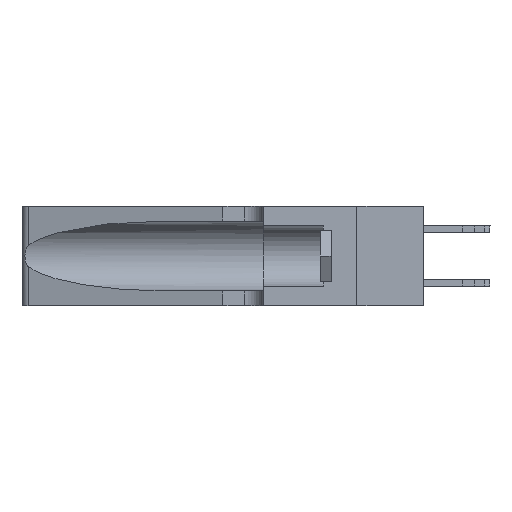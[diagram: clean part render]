
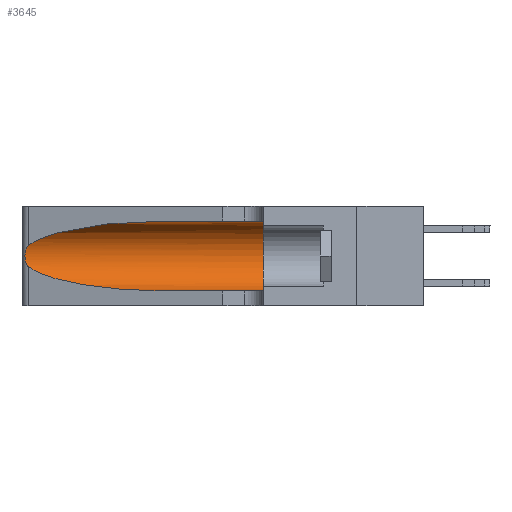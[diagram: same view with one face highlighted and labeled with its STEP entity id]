
A CAD part, left-side view. The second image highlights one B-rep face of the part: STEP entity #3645.
In plain terms, the highlighted cylindrical face has radius 3.308 mm (diameter 6.617 mm), a partial arc.
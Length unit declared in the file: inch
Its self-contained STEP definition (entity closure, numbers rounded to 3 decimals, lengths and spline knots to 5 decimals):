
#310 = AXIS2_PLACEMENT_3D ( 'NONE', #10544, #16618, #24730 ) ;
#458 = CARTESIAN_POINT ( 'NONE',  ( 0.1305, 1.61858, 0.185 ) ) ;
#866 = ORIENTED_EDGE ( 'NONE', *, *, #23540, .T. ) ;
#966 = ORIENTED_EDGE ( 'NONE', *, *, #2103, .T. ) ;
#1143 = DIRECTION ( 'NONE',  ( 0., -1., 0. ) ) ;
#1354 = VERTEX_POINT ( 'NONE', #17945 ) ;
#1531 = CARTESIAN_POINT ( 'NONE',  ( 0.25854, 1.2359, 0.20912 ) ) ;
#2103 = EDGE_CURVE ( 'NONE', #21061, #22605, #16214, .T. ) ;
#3618 = LINE ( 'NONE', #13587, #15790 ) ;
#3645 = ADVANCED_FACE ( 'NONE', ( #9608 ), #23735, .F. ) ;
#4130 = DIRECTION ( 'NONE',  ( 0., -1., 0. ) ) ;
#4241 = ORIENTED_EDGE ( 'NONE', *, *, #9522, .T. ) ;
#5245 = EDGE_CURVE ( 'NONE', #1354, #21061, #9823, .T. ) ;
#5681 = CARTESIAN_POINT ( 'NONE',  ( 0.26075, 1.23896, 0.178 ) ) ;
#5863 = CARTESIAN_POINT ( 'NONE',  ( 0.25487, 1.22718, 0.14631 ) ) ;
#6300 = EDGE_CURVE ( 'NONE', #1354, #17870, #21706, .T. ) ;
#6306 = CARTESIAN_POINT ( 'NONE',  ( 0.25487, 1.22718, 0.14631 ) ) ;
#7753 = CARTESIAN_POINT ( 'NONE',  ( 0.25639, 1.23186, 0.15144 ) ) ;
#7998 = CARTESIAN_POINT ( 'NONE',  ( 0.25555, 1.22993, 0.14849 ) ) ;
#9522 = EDGE_CURVE ( 'NONE', #11176, #26147, #3618, .T. ) ;
#9608 = FACE_OUTER_BOUND ( 'NONE', #21091, .T. ) ;
#9728 = CARTESIAN_POINT ( 'NONE',  ( 0.26018, 1.23835, 0.19895 ) ) ;
#9806 = CARTESIAN_POINT ( 'NONE',  ( 0.26017, 1.23833, 0.17102 ) ) ;
#9823 =( BOUNDED_CURVE ( )  B_SPLINE_CURVE ( 3, ( #18706, #22653, #14734, #20952 ),
 .UNSPECIFIED., .F., .T. ) 
 B_SPLINE_CURVE_WITH_KNOTS ( ( 4, 4 ),
 ( 1.5708, 2.84003 ),
 .UNSPECIFIED. ) 
 CURVE ( )  GEOMETRIC_REPRESENTATION_ITEM ( )  RATIONAL_B_SPLINE_CURVE ( ( 1., 0.87, 0.87, 1. ) ) 
 REPRESENTATION_ITEM ( '' )  );
#9943 = ORIENTED_EDGE ( 'NONE', *, *, #5245, .T. ) ;
#10544 = CARTESIAN_POINT ( 'NONE',  ( 0.1305, 0.35, 0.185 ) ) ;
#11127 =( BOUNDED_CURVE ( )  B_SPLINE_CURVE ( 3, ( #12026, #26406, #17936, #11847 ),
 .UNSPECIFIED., .F., .T. ) 
 B_SPLINE_CURVE_WITH_KNOTS ( ( 4, 4 ),
 ( 3.44316, 4.71239 ),
 .UNSPECIFIED. ) 
 CURVE ( )  GEOMETRIC_REPRESENTATION_ITEM ( )  RATIONAL_B_SPLINE_CURVE ( ( 1., 0.87, 0.87, 1. ) ) 
 REPRESENTATION_ITEM ( '' )  );
#11176 = VERTEX_POINT ( 'NONE', #25803 ) ;
#11610 = CIRCLE ( 'NONE', #310, 0.13025 ) ;
#11847 = CARTESIAN_POINT ( 'NONE',  ( 0.1305, 0.72297, 0.05475 ) ) ;
#12026 = CARTESIAN_POINT ( 'NONE',  ( 0.25487, 1.22718, 0.14631 ) ) ;
#12349 = CARTESIAN_POINT ( 'NONE',  ( 0.1305, 1.61858, 0.31525 ) ) ;
#12476 = ORIENTED_EDGE ( 'NONE', *, *, #6300, .F. ) ;
#12758 = ORIENTED_EDGE ( 'NONE', *, *, #17728, .F. ) ;
#13587 = CARTESIAN_POINT ( 'NONE',  ( 0.1305, 1.61858, 0.05475 ) ) ;
#13684 = VECTOR ( 'NONE', #4130, 39.37008 ) ;
#14734 = CARTESIAN_POINT ( 'NONE',  ( 0.2373, 1.15595, 0.28018 ) ) ;
#15790 = VECTOR ( 'NONE', #26047, 39.37008 ) ;
#16214 = B_SPLINE_CURVE_WITH_KNOTS ( 'NONE', 3,
 ( #17940, #22353, #24168, #20100, #1531, #9728, #18211, #5681, #9806, #20015, #16239, #7753, #7998, #5863 ),
 .UNSPECIFIED., .F., .F.,
 ( 4, 2, 2, 2, 2, 2, 4 ),
 ( 0., 0.00027, 0.00053, 0.00107, 0.0016, 0.00187, 0.00214 ),
 .UNSPECIFIED. ) ;
#16239 = CARTESIAN_POINT ( 'NONE',  ( 0.25789, 1.23486, 0.15765 ) ) ;
#16428 = AXIS2_PLACEMENT_3D ( 'NONE', #458, #1143, #19798 ) ;
#16618 = DIRECTION ( 'NONE',  ( 0., 1., 0. ) ) ;
#17728 = EDGE_CURVE ( 'NONE', #17870, #26147, #11610, .T. ) ;
#17870 = VERTEX_POINT ( 'NONE', #24843 ) ;
#17936 = CARTESIAN_POINT ( 'NONE',  ( 0.18966, 0.96281, 0.05475 ) ) ;
#17940 = CARTESIAN_POINT ( 'NONE',  ( 0.25487, 1.22718, 0.22369 ) ) ;
#17945 = CARTESIAN_POINT ( 'NONE',  ( 0.1305, 0.72297, 0.31525 ) ) ;
#18211 = CARTESIAN_POINT ( 'NONE',  ( 0.26075, 1.23896, 0.19203 ) ) ;
#18706 = CARTESIAN_POINT ( 'NONE',  ( 0.1305, 0.72297, 0.31525 ) ) ;
#19712 = CARTESIAN_POINT ( 'NONE',  ( 0.1305, 0.35, 0.05475 ) ) ;
#19798 = DIRECTION ( 'NONE',  ( 0., 0., -1. ) ) ;
#20015 = CARTESIAN_POINT ( 'NONE',  ( 0.25856, 1.23593, 0.16098 ) ) ;
#20100 = CARTESIAN_POINT ( 'NONE',  ( 0.25787, 1.23484, 0.2124 ) ) ;
#20952 = CARTESIAN_POINT ( 'NONE',  ( 0.25487, 1.22718, 0.22369 ) ) ;
#21061 = VERTEX_POINT ( 'NONE', #23714 ) ;
#21091 = EDGE_LOOP ( 'NONE', ( #9943, #966, #866, #4241, #12758, #12476 ) ) ;
#21706 = LINE ( 'NONE', #12349, #13684 ) ;
#22353 = CARTESIAN_POINT ( 'NONE',  ( 0.25555, 1.22994, 0.2215 ) ) ;
#22605 = VERTEX_POINT ( 'NONE', #6306 ) ;
#22653 = CARTESIAN_POINT ( 'NONE',  ( 0.18966, 0.96281, 0.31525 ) ) ;
#23540 = EDGE_CURVE ( 'NONE', #22605, #11176, #11127, .T. ) ;
#23714 = CARTESIAN_POINT ( 'NONE',  ( 0.25487, 1.22718, 0.22369 ) ) ;
#23735 = CYLINDRICAL_SURFACE ( 'NONE', #16428, 0.13025 ) ;
#24168 = CARTESIAN_POINT ( 'NONE',  ( 0.25639, 1.23184, 0.21858 ) ) ;
#24730 = DIRECTION ( 'NONE',  ( 0., 0., 1. ) ) ;
#24843 = CARTESIAN_POINT ( 'NONE',  ( 0.1305, 0.35, 0.31525 ) ) ;
#25803 = CARTESIAN_POINT ( 'NONE',  ( 0.1305, 0.72297, 0.05475 ) ) ;
#26047 = DIRECTION ( 'NONE',  ( 0., -1., 0. ) ) ;
#26147 = VERTEX_POINT ( 'NONE', #19712 ) ;
#26406 = CARTESIAN_POINT ( 'NONE',  ( 0.2373, 1.15595, 0.08982 ) ) ;
